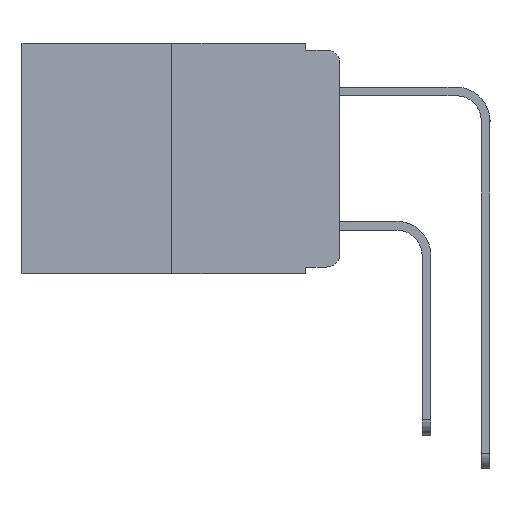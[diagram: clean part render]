
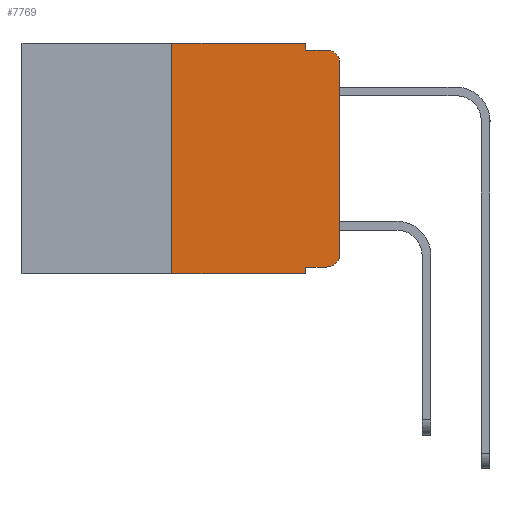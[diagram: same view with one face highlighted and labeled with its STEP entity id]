
A CAD part, left-side view. The second image highlights one B-rep face of the part: STEP entity #7769.
In plain terms, the highlighted planar face has unit normal (-1, 0, 0).
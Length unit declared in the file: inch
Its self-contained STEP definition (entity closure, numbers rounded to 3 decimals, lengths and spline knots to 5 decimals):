
#415 = ORIENTED_EDGE ( 'NONE', *, *, #17014, .T. ) ;
#431 = CIRCLE ( 'NONE', #22308, 0.02 ) ;
#1170 = LINE ( 'NONE', #12037, #16548 ) ;
#1242 = CARTESIAN_POINT ( 'NONE',  ( 0., 0.051, 0. ) ) ;
#1883 = VERTEX_POINT ( 'NONE', #12013 ) ;
#1914 = CARTESIAN_POINT ( 'NONE',  ( 0., 0.051, -0.333 ) ) ;
#2000 = LINE ( 'NONE', #5494, #11746 ) ;
#2320 = VERTEX_POINT ( 'NONE', #18873 ) ;
#2464 = VERTEX_POINT ( 'NONE', #3541 ) ;
#2773 = PLANE ( 'NONE',  #7850 ) ;
#3071 = CARTESIAN_POINT ( 'NONE',  ( 0., 0.051, 0. ) ) ;
#3147 = VERTEX_POINT ( 'NONE', #12573 ) ;
#3541 = CARTESIAN_POINT ( 'NONE',  ( 0., 0., -0.313 ) ) ;
#4111 = ORIENTED_EDGE ( 'NONE', *, *, #14156, .T. ) ;
#4296 = AXIS2_PLACEMENT_3D ( 'NONE', #10530, #23631, #12465 ) ;
#4418 = ORIENTED_EDGE ( 'NONE', *, *, #19217, .F. ) ;
#4477 = EDGE_LOOP ( 'NONE', ( #23060, #20477, #6555, #19045, #21652, #4418, #415, #11415, #22522, #4111 ) ) ;
#4482 = LINE ( 'NONE', #1242, #18540 ) ;
#5494 = CARTESIAN_POINT ( 'NONE',  ( 0., 0.051, -0.01 ) ) ;
#6280 = VERTEX_POINT ( 'NONE', #17587 ) ;
#6407 = FACE_OUTER_BOUND ( 'NONE', #4477, .T. ) ;
#6555 = ORIENTED_EDGE ( 'NONE', *, *, #21679, .F. ) ;
#7517 = DIRECTION ( 'NONE',  ( 0., 0., -1. ) ) ;
#7769 = ADVANCED_FACE ( 'NONE', ( #6407 ), #2773, .F. ) ;
#7819 = VERTEX_POINT ( 'NONE', #20165 ) ;
#7824 = CARTESIAN_POINT ( 'NONE',  ( 0., 0.02, -0.313 ) ) ;
#7850 = AXIS2_PLACEMENT_3D ( 'NONE', #8693, #23716, #12541 ) ;
#8379 = CARTESIAN_POINT ( 'NONE',  ( 0., 0.473, -0.343 ) ) ;
#8459 = CIRCLE ( 'NONE', #4296, 0.02 ) ;
#8527 = CARTESIAN_POINT ( 'NONE',  ( 0., 0., -0.03 ) ) ;
#8638 = CARTESIAN_POINT ( 'NONE',  ( 0., 0., 0. ) ) ;
#8693 = CARTESIAN_POINT ( 'NONE',  ( 0., 0.473, 0. ) ) ;
#8764 = VERTEX_POINT ( 'NONE', #19083 ) ;
#9740 = DIRECTION ( 'NONE',  ( 0., 0., -1. ) ) ;
#10215 = VERTEX_POINT ( 'NONE', #10731 ) ;
#10530 = CARTESIAN_POINT ( 'NONE',  ( 0., 0.02, -0.03 ) ) ;
#10677 = VECTOR ( 'NONE', #7517, 39.37008 ) ;
#10731 = CARTESIAN_POINT ( 'NONE',  ( 0., 0.02, -0.333 ) ) ;
#11415 = ORIENTED_EDGE ( 'NONE', *, *, #17970, .F. ) ;
#11746 = VECTOR ( 'NONE', #20685, 39.37008 ) ;
#11833 = EDGE_CURVE ( 'NONE', #8764, #21514, #1170, .T. ) ;
#11967 = VECTOR ( 'NONE', #13519, 39.37008 ) ;
#12013 = CARTESIAN_POINT ( 'NONE',  ( 0., 0.051, -0.01 ) ) ;
#12037 = CARTESIAN_POINT ( 'NONE',  ( 0., 0.473, 0. ) ) ;
#12424 = LINE ( 'NONE', #20711, #21776 ) ;
#12465 = DIRECTION ( 'NONE',  ( 0., 0., -1. ) ) ;
#12541 = DIRECTION ( 'NONE',  ( 0., 0., -1. ) ) ;
#12573 = CARTESIAN_POINT ( 'NONE',  ( 0., 0.02, -0.01 ) ) ;
#13519 = DIRECTION ( 'NONE',  ( 0., -1., 0. ) ) ;
#13825 = DIRECTION ( 'NONE',  ( 0., -1., 0. ) ) ;
#14156 = EDGE_CURVE ( 'NONE', #10215, #2464, #431, .T. ) ;
#14827 = DIRECTION ( 'NONE',  ( 0., 0., -1. ) ) ;
#15415 = EDGE_CURVE ( 'NONE', #7819, #10215, #21896, .T. ) ;
#15699 = LINE ( 'NONE', #22569, #10677 ) ;
#15705 = VERTEX_POINT ( 'NONE', #8527 ) ;
#16548 = VECTOR ( 'NONE', #13825, 39.37008 ) ;
#16952 = LINE ( 'NONE', #8379, #17546 ) ;
#17014 = EDGE_CURVE ( 'NONE', #6280, #2320, #16952, .T. ) ;
#17546 = VECTOR ( 'NONE', #21559, 39.37008 ) ;
#17587 = CARTESIAN_POINT ( 'NONE',  ( 0., 0.25, -0.343 ) ) ;
#17970 = EDGE_CURVE ( 'NONE', #7819, #2320, #15699, .T. ) ;
#18540 = VECTOR ( 'NONE', #14827, 39.37008 ) ;
#18873 = CARTESIAN_POINT ( 'NONE',  ( 0., 0.051, -0.343 ) ) ;
#19045 = ORIENTED_EDGE ( 'NONE', *, *, #20442, .F. ) ;
#19056 = VECTOR ( 'NONE', #19972, 39.37008 ) ;
#19083 = CARTESIAN_POINT ( 'NONE',  ( 0., 0.25, 0. ) ) ;
#19217 = EDGE_CURVE ( 'NONE', #6280, #8764, #12424, .T. ) ;
#19972 = DIRECTION ( 'NONE',  ( 0., 0., 1. ) ) ;
#20165 = CARTESIAN_POINT ( 'NONE',  ( 0., 0.051, -0.333 ) ) ;
#20442 = EDGE_CURVE ( 'NONE', #21514, #1883, #4482, .T. ) ;
#20477 = ORIENTED_EDGE ( 'NONE', *, *, #22902, .T. ) ;
#20685 = DIRECTION ( 'NONE',  ( 0., -1., 0. ) ) ;
#20711 = CARTESIAN_POINT ( 'NONE',  ( 0., 0.25, 0. ) ) ;
#21021 = DIRECTION ( 'NONE',  ( -1., 0., 0. ) ) ;
#21514 = VERTEX_POINT ( 'NONE', #3071 ) ;
#21559 = DIRECTION ( 'NONE',  ( 0., -1., 0. ) ) ;
#21652 = ORIENTED_EDGE ( 'NONE', *, *, #11833, .F. ) ;
#21679 = EDGE_CURVE ( 'NONE', #1883, #3147, #2000, .T. ) ;
#21776 = VECTOR ( 'NONE', #24416, 39.37008 ) ;
#21896 = LINE ( 'NONE', #1914, #11967 ) ;
#22308 = AXIS2_PLACEMENT_3D ( 'NONE', #7824, #21021, #9740 ) ;
#22522 = ORIENTED_EDGE ( 'NONE', *, *, #15415, .T. ) ;
#22569 = CARTESIAN_POINT ( 'NONE',  ( 0., 0.051, 0. ) ) ;
#22902 = EDGE_CURVE ( 'NONE', #15705, #3147, #8459, .T. ) ;
#23060 = ORIENTED_EDGE ( 'NONE', *, *, #24149, .T. ) ;
#23374 = LINE ( 'NONE', #8638, #19056 ) ;
#23631 = DIRECTION ( 'NONE',  ( -1., 0., 0. ) ) ;
#23716 = DIRECTION ( 'NONE',  ( 1., 0., 0. ) ) ;
#24149 = EDGE_CURVE ( 'NONE', #2464, #15705, #23374, .T. ) ;
#24416 = DIRECTION ( 'NONE',  ( 0., 0., 1. ) ) ;
